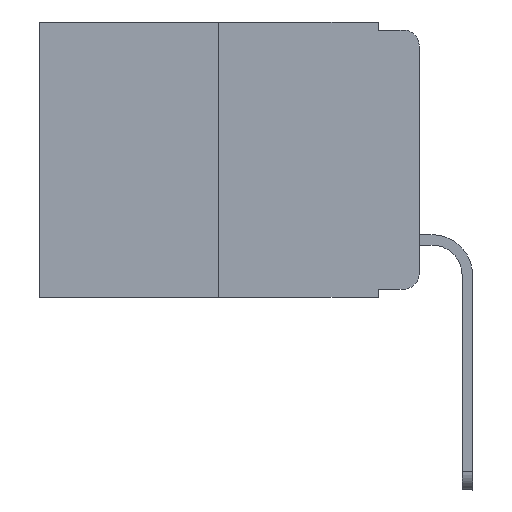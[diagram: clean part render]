
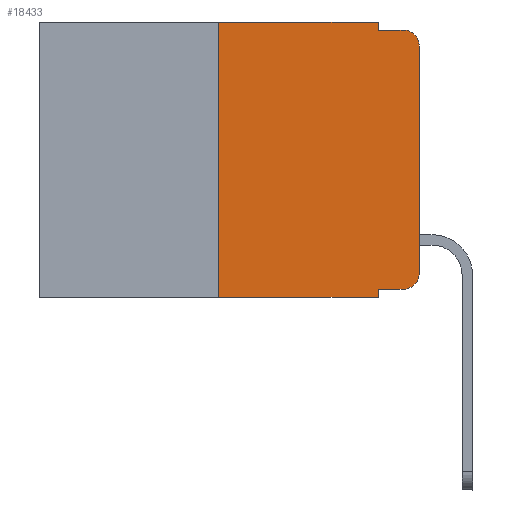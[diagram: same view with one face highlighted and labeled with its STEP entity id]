
A CAD part, left-side view. The second image highlights one B-rep face of the part: STEP entity #18433.
In plain terms, the highlighted planar face has unit normal (-1, 0, 0).
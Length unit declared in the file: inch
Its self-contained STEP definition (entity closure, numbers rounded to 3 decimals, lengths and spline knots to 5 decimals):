
#426 = DIRECTION ( 'NONE',  ( -1., 0., 0. ) ) ;
#714 = DIRECTION ( 'NONE',  ( 0., 0., 1. ) ) ;
#1001 = ORIENTED_EDGE ( 'NONE', *, *, #18089, .T. ) ;
#1119 = VECTOR ( 'NONE', #18718, 39.37008 ) ;
#1318 = VECTOR ( 'NONE', #2488, 39.37008 ) ;
#1509 = VERTEX_POINT ( 'NONE', #13968 ) ;
#1874 = LINE ( 'NONE', #18516, #1119 ) ;
#2130 = CARTESIAN_POINT ( 'NONE',  ( 0., 0.051, 0. ) ) ;
#2131 = CARTESIAN_POINT ( 'NONE',  ( 0., 0.051, 0. ) ) ;
#2488 = DIRECTION ( 'NONE',  ( 0., -1., 0. ) ) ;
#2572 = VECTOR ( 'NONE', #15813, 39.37008 ) ;
#2663 = VECTOR ( 'NONE', #11017, 39.37008 ) ;
#2883 = EDGE_CURVE ( 'NONE', #12349, #16708, #5497, .T. ) ;
#2977 = EDGE_CURVE ( 'NONE', #6847, #1509, #9795, .T. ) ;
#3043 = CIRCLE ( 'NONE', #14190, 0.02 ) ;
#3090 = AXIS2_PLACEMENT_3D ( 'NONE', #5434, #13113, #11974 ) ;
#3451 = PLANE ( 'NONE',  #3090 ) ;
#3569 = VERTEX_POINT ( 'NONE', #11857 ) ;
#3771 = EDGE_CURVE ( 'NONE', #3569, #16251, #3865, .T. ) ;
#3785 = AXIS2_PLACEMENT_3D ( 'NONE', #9503, #426, #15277 ) ;
#3865 = LINE ( 'NONE', #5054, #2572 ) ;
#3936 = LINE ( 'NONE', #16190, #13601 ) ;
#4172 = DIRECTION ( 'NONE',  ( 0., 0., -1. ) ) ;
#4247 = VERTEX_POINT ( 'NONE', #2130 ) ;
#4411 = VECTOR ( 'NONE', #714, 39.37008 ) ;
#4738 = ORIENTED_EDGE ( 'NONE', *, *, #14106, .F. ) ;
#5054 = CARTESIAN_POINT ( 'NONE',  ( 0., 0.25, 0. ) ) ;
#5160 = ORIENTED_EDGE ( 'NONE', *, *, #16865, .T. ) ;
#5355 = EDGE_CURVE ( 'NONE', #14166, #16911, #10828, .T. ) ;
#5396 = CARTESIAN_POINT ( 'NONE',  ( 0., 0.051, -0.333 ) ) ;
#5434 = CARTESIAN_POINT ( 'NONE',  ( 0., 0.473, 0. ) ) ;
#5497 = LINE ( 'NONE', #11009, #4411 ) ;
#6439 = EDGE_CURVE ( 'NONE', #16251, #4247, #8671, .T. ) ;
#6590 = VECTOR ( 'NONE', #8216, 39.37008 ) ;
#6683 = ORIENTED_EDGE ( 'NONE', *, *, #2883, .T. ) ;
#6847 = VERTEX_POINT ( 'NONE', #12161 ) ;
#7106 = DIRECTION ( 'NONE',  ( 0., 0., -1. ) ) ;
#7786 = EDGE_LOOP ( 'NONE', ( #6683, #5160, #10172, #4738, #10751, #11903, #11866, #11080, #11655, #1001 ) ) ;
#8216 = DIRECTION ( 'NONE',  ( 0., 0., -1. ) ) ;
#8510 = CARTESIAN_POINT ( 'NONE',  ( 0., 0.051, -0.01 ) ) ;
#8671 = LINE ( 'NONE', #14741, #1318 ) ;
#8685 = DIRECTION ( 'NONE',  ( 0., -1., 0. ) ) ;
#8912 = CARTESIAN_POINT ( 'NONE',  ( 0., 0., -0.03 ) ) ;
#9503 = CARTESIAN_POINT ( 'NONE',  ( 0., 0.02, -0.03 ) ) ;
#9795 = LINE ( 'NONE', #5396, #13655 ) ;
#9834 = FACE_OUTER_BOUND ( 'NONE', #7786, .T. ) ;
#9875 = EDGE_CURVE ( 'NONE', #3569, #13313, #1874, .T. ) ;
#10172 = ORIENTED_EDGE ( 'NONE', *, *, #5355, .F. ) ;
#10751 = ORIENTED_EDGE ( 'NONE', *, *, #6439, .F. ) ;
#10828 = LINE ( 'NONE', #16889, #2663 ) ;
#11009 = CARTESIAN_POINT ( 'NONE',  ( 0., 0., 0. ) ) ;
#11017 = DIRECTION ( 'NONE',  ( 0., -1., 0. ) ) ;
#11080 = ORIENTED_EDGE ( 'NONE', *, *, #14214, .F. ) ;
#11655 = ORIENTED_EDGE ( 'NONE', *, *, #2977, .T. ) ;
#11857 = CARTESIAN_POINT ( 'NONE',  ( 0., 0.25, -0.343 ) ) ;
#11866 = ORIENTED_EDGE ( 'NONE', *, *, #9875, .T. ) ;
#11903 = ORIENTED_EDGE ( 'NONE', *, *, #3771, .F. ) ;
#11974 = DIRECTION ( 'NONE',  ( 0., 0., -1. ) ) ;
#12161 = CARTESIAN_POINT ( 'NONE',  ( 0., 0.051, -0.333 ) ) ;
#12349 = VERTEX_POINT ( 'NONE', #14117 ) ;
#13018 = CIRCLE ( 'NONE', #3785, 0.02 ) ;
#13113 = DIRECTION ( 'NONE',  ( 1., 0., 0. ) ) ;
#13313 = VERTEX_POINT ( 'NONE', #19242 ) ;
#13601 = VECTOR ( 'NONE', #7106, 39.37008 ) ;
#13655 = VECTOR ( 'NONE', #8685, 39.37008 ) ;
#13968 = CARTESIAN_POINT ( 'NONE',  ( 0., 0.02, -0.333 ) ) ;
#14106 = EDGE_CURVE ( 'NONE', #4247, #14166, #18786, .T. ) ;
#14117 = CARTESIAN_POINT ( 'NONE',  ( 0., 0., -0.313 ) ) ;
#14166 = VERTEX_POINT ( 'NONE', #8510 ) ;
#14190 = AXIS2_PLACEMENT_3D ( 'NONE', #17829, #16414, #4172 ) ;
#14214 = EDGE_CURVE ( 'NONE', #6847, #13313, #3936, .T. ) ;
#14249 = CARTESIAN_POINT ( 'NONE',  ( 0., 0.25, 0. ) ) ;
#14741 = CARTESIAN_POINT ( 'NONE',  ( 0., 0.473, 0. ) ) ;
#15277 = DIRECTION ( 'NONE',  ( 0., 0., -1. ) ) ;
#15373 = CARTESIAN_POINT ( 'NONE',  ( 0., 0.02, -0.01 ) ) ;
#15813 = DIRECTION ( 'NONE',  ( 0., 0., 1. ) ) ;
#16190 = CARTESIAN_POINT ( 'NONE',  ( 0., 0.051, 0. ) ) ;
#16251 = VERTEX_POINT ( 'NONE', #14249 ) ;
#16414 = DIRECTION ( 'NONE',  ( -1., 0., 0. ) ) ;
#16708 = VERTEX_POINT ( 'NONE', #8912 ) ;
#16865 = EDGE_CURVE ( 'NONE', #16708, #16911, #13018, .T. ) ;
#16889 = CARTESIAN_POINT ( 'NONE',  ( 0., 0.051, -0.01 ) ) ;
#16911 = VERTEX_POINT ( 'NONE', #15373 ) ;
#17829 = CARTESIAN_POINT ( 'NONE',  ( 0., 0.02, -0.313 ) ) ;
#18089 = EDGE_CURVE ( 'NONE', #1509, #12349, #3043, .T. ) ;
#18433 = ADVANCED_FACE ( 'NONE', ( #9834 ), #3451, .F. ) ;
#18516 = CARTESIAN_POINT ( 'NONE',  ( 0., 0.473, -0.343 ) ) ;
#18718 = DIRECTION ( 'NONE',  ( 0., -1., 0. ) ) ;
#18786 = LINE ( 'NONE', #2131, #6590 ) ;
#19242 = CARTESIAN_POINT ( 'NONE',  ( 0., 0.051, -0.343 ) ) ;
